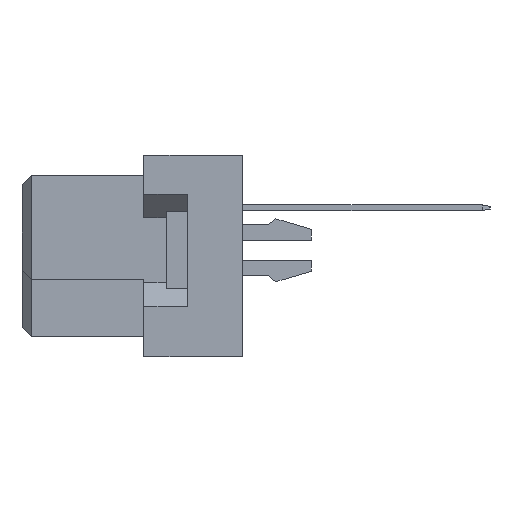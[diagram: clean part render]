
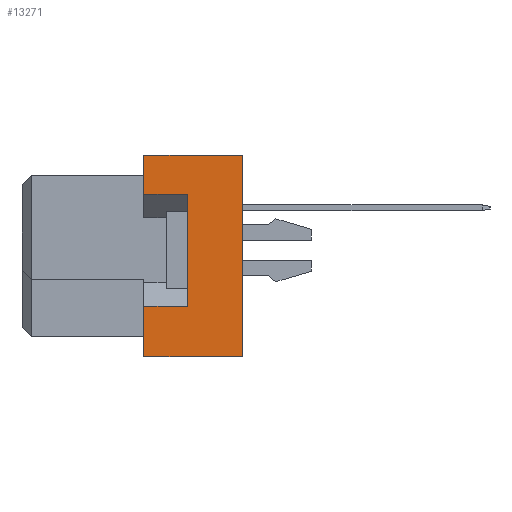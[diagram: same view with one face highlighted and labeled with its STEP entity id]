
A CAD part, left-side view. The second image highlights one B-rep face of the part: STEP entity #13271.
In plain terms, the highlighted planar face has unit normal (-1, 0, 0).
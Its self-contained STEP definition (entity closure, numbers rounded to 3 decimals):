
#112 = EDGE_CURVE ( 'NONE', #26957, #13954, #6828, .T. ) ;
#578 = ORIENTED_EDGE ( 'NONE', *, *, #112, .T. ) ;
#702 = CARTESIAN_POINT ( 'NONE',  ( -47.5, -8.7, 3.25 ) ) ;
#1098 = EDGE_CURVE ( 'NONE', #17614, #38562, #6774, .T. ) ;
#1372 = ORIENTED_EDGE ( 'NONE', *, *, #10316, .F. ) ;
#1411 = ORIENTED_EDGE ( 'NONE', *, *, #1098, .F. ) ;
#1556 = VERTEX_POINT ( 'NONE', #3218 ) ;
#3061 = EDGE_CURVE ( 'NONE', #26957, #32912, #33828, .T. ) ;
#3218 = CARTESIAN_POINT ( 'NONE',  ( -47.5, -6.4, -5.3 ) ) ;
#4367 = LINE ( 'NONE', #34078, #13672 ) ;
#4489 = LINE ( 'NONE', #26111, #7575 ) ;
#5104 = ORIENTED_EDGE ( 'NONE', *, *, #38185, .T. ) ;
#6402 = EDGE_CURVE ( 'NONE', #15230, #1556, #13452, .T. ) ;
#6677 = CARTESIAN_POINT ( 'NONE',  ( -47.5, -6.4, 3.25 ) ) ;
#6774 = LINE ( 'NONE', #21932, #36474 ) ;
#6807 = DIRECTION ( 'NONE',  ( 0., 1., 0. ) ) ;
#6828 = LINE ( 'NONE', #7624, #16258 ) ;
#7575 = VECTOR ( 'NONE', #19654, 1000. ) ;
#7624 = CARTESIAN_POINT ( 'NONE',  ( -47.5, -8.7, -2.65 ) ) ;
#8691 = ORIENTED_EDGE ( 'NONE', *, *, #3061, .F. ) ;
#9051 = ORIENTED_EDGE ( 'NONE', *, *, #6402, .F. ) ;
#10212 = ORIENTED_EDGE ( 'NONE', *, *, #13572, .F. ) ;
#10280 = DIRECTION ( 'NONE',  ( 0., 0., 1. ) ) ;
#10316 = EDGE_CURVE ( 'NONE', #1556, #13954, #4367, .T. ) ;
#10485 = DIRECTION ( 'NONE',  ( 0., 1., 0. ) ) ;
#11471 = CARTESIAN_POINT ( 'NONE',  ( -47.5, -11.6, 5.3 ) ) ;
#12323 = LINE ( 'NONE', #18441, #27609 ) ;
#12803 = DIRECTION ( 'NONE',  ( 0., 0., 1. ) ) ;
#12911 = DIRECTION ( 'NONE',  ( 0., 0., 1. ) ) ;
#13271 = ADVANCED_FACE ( 'NONE', ( #22397 ), #20239, .T. ) ;
#13452 = LINE ( 'NONE', #31549, #26491 ) ;
#13572 = EDGE_CURVE ( 'NONE', #32912, #17614, #24909, .T. ) ;
#13672 = VECTOR ( 'NONE', #10280, 1000. ) ;
#13954 = VERTEX_POINT ( 'NONE', #36053 ) ;
#14698 = VECTOR ( 'NONE', #12803, 1000. ) ;
#15230 = VERTEX_POINT ( 'NONE', #24690 ) ;
#16258 = VECTOR ( 'NONE', #37130, 1000. ) ;
#17614 = VERTEX_POINT ( 'NONE', #6677 ) ;
#18253 = CARTESIAN_POINT ( 'NONE',  ( -47.5, -8.7, 3.25 ) ) ;
#18441 = CARTESIAN_POINT ( 'NONE',  ( -47.5, -11.6, 5.3 ) ) ;
#18799 = DIRECTION ( 'NONE',  ( 0., 0., 1. ) ) ;
#19654 = DIRECTION ( 'NONE',  ( 0., 1., 0. ) ) ;
#20106 = AXIS2_PLACEMENT_3D ( 'NONE', #28687, #37932, #22603 ) ;
#20239 = PLANE ( 'NONE',  #20106 ) ;
#21932 = CARTESIAN_POINT ( 'NONE',  ( -47.5, -6.4, -5.3 ) ) ;
#22397 = FACE_OUTER_BOUND ( 'NONE', #33520, .T. ) ;
#22603 = DIRECTION ( 'NONE',  ( 0., 0., 1. ) ) ;
#24690 = CARTESIAN_POINT ( 'NONE',  ( -47.5, -11.6, -5.3 ) ) ;
#24909 = LINE ( 'NONE', #18253, #33897 ) ;
#24934 = EDGE_CURVE ( 'NONE', #15230, #25642, #12323, .T. ) ;
#25642 = VERTEX_POINT ( 'NONE', #11471 ) ;
#26111 = CARTESIAN_POINT ( 'NONE',  ( -47.5, -11.6, 5.3 ) ) ;
#26203 = ORIENTED_EDGE ( 'NONE', *, *, #24934, .T. ) ;
#26491 = VECTOR ( 'NONE', #10485, 1000. ) ;
#26957 = VERTEX_POINT ( 'NONE', #35865 ) ;
#27609 = VECTOR ( 'NONE', #12911, 1000. ) ;
#28687 = CARTESIAN_POINT ( 'NONE',  ( -47.5, -11.6, 5.3 ) ) ;
#31549 = CARTESIAN_POINT ( 'NONE',  ( -47.5, -11.6, -5.3 ) ) ;
#32912 = VERTEX_POINT ( 'NONE', #702 ) ;
#33520 = EDGE_LOOP ( 'NONE', ( #578, #1372, #9051, #26203, #5104, #1411, #10212, #8691 ) ) ;
#33828 = LINE ( 'NONE', #36205, #14698 ) ;
#33897 = VECTOR ( 'NONE', #6807, 1000. ) ;
#34078 = CARTESIAN_POINT ( 'NONE',  ( -47.5, -6.4, -5.3 ) ) ;
#35865 = CARTESIAN_POINT ( 'NONE',  ( -47.5, -8.7, -2.65 ) ) ;
#36053 = CARTESIAN_POINT ( 'NONE',  ( -47.5, -6.4, -2.65 ) ) ;
#36205 = CARTESIAN_POINT ( 'NONE',  ( -47.5, -8.7, -2.65 ) ) ;
#36474 = VECTOR ( 'NONE', #18799, 1000. ) ;
#37130 = DIRECTION ( 'NONE',  ( 0., 1., 0. ) ) ;
#37932 = DIRECTION ( 'NONE',  ( -1., 0., 0. ) ) ;
#38055 = CARTESIAN_POINT ( 'NONE',  ( -47.5, -6.4, 5.3 ) ) ;
#38185 = EDGE_CURVE ( 'NONE', #25642, #38562, #4489, .T. ) ;
#38562 = VERTEX_POINT ( 'NONE', #38055 ) ;
